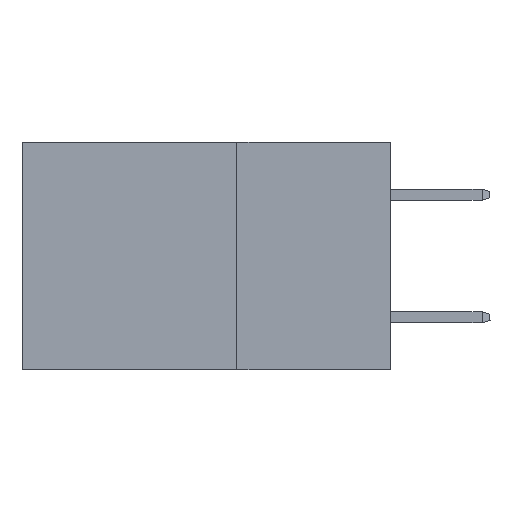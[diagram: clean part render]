
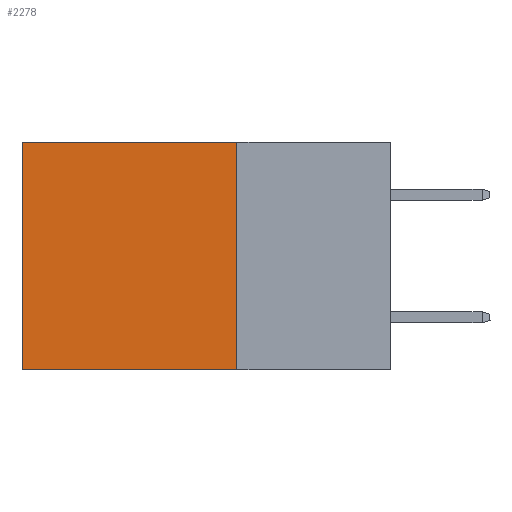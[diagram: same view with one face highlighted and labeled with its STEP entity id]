
A CAD part, left-side view. The second image highlights one B-rep face of the part: STEP entity #2278.
In plain terms, the highlighted planar face has unit normal (-1, 0, 0).
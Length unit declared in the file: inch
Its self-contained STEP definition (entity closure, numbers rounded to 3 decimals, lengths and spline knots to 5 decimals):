
#25 = LINE ( 'NONE', #17002, #10914 ) ;
#1154 = DIRECTION ( 'NONE',  ( 0., 1., 0. ) ) ;
#2278 = ADVANCED_FACE ( 'NONE', ( #18125 ), #16090, .F. ) ;
#2668 = CARTESIAN_POINT ( 'NONE',  ( 0.2875, 0.25, 0. ) ) ;
#3081 = VECTOR ( 'NONE', #5774, 39.37008 ) ;
#5774 = DIRECTION ( 'NONE',  ( 0., 0., -1. ) ) ;
#6467 = VECTOR ( 'NONE', #13831, 39.37008 ) ;
#6862 = VERTEX_POINT ( 'NONE', #9644 ) ;
#7752 = VERTEX_POINT ( 'NONE', #12504 ) ;
#8001 = LINE ( 'NONE', #8198, #10917 ) ;
#8198 = CARTESIAN_POINT ( 'NONE',  ( 0.2875, 0.25, 0. ) ) ;
#8431 = DIRECTION ( 'NONE',  ( 0., 1., 0. ) ) ;
#9117 = EDGE_CURVE ( 'NONE', #13216, #7752, #13255, .T. ) ;
#9223 = EDGE_CURVE ( 'NONE', #13216, #11601, #8001, .T. ) ;
#9644 = CARTESIAN_POINT ( 'NONE',  ( 0.2875, 0.6, -0.37 ) ) ;
#10241 = DIRECTION ( 'NONE',  ( 0., 0., -1. ) ) ;
#10796 = AXIS2_PLACEMENT_3D ( 'NONE', #14763, #11859, #10241 ) ;
#10914 = VECTOR ( 'NONE', #1154, 39.37008 ) ;
#10917 = VECTOR ( 'NONE', #8431, 39.37008 ) ;
#11028 = CARTESIAN_POINT ( 'NONE',  ( 0.2875, 0.25, 0. ) ) ;
#11566 = EDGE_LOOP ( 'NONE', ( #13420, #16666, #16898, #16736 ) ) ;
#11601 = VERTEX_POINT ( 'NONE', #13120 ) ;
#11859 = DIRECTION ( 'NONE',  ( 1., 0., 0. ) ) ;
#12504 = CARTESIAN_POINT ( 'NONE',  ( 0.2875, 0.25, -0.37 ) ) ;
#13120 = CARTESIAN_POINT ( 'NONE',  ( 0.2875, 0.6, 0. ) ) ;
#13216 = VERTEX_POINT ( 'NONE', #2668 ) ;
#13255 = LINE ( 'NONE', #11028, #6467 ) ;
#13420 = ORIENTED_EDGE ( 'NONE', *, *, #15662, .T. ) ;
#13831 = DIRECTION ( 'NONE',  ( 0., 0., -1. ) ) ;
#14763 = CARTESIAN_POINT ( 'NONE',  ( 0.2875, 0.25, 0. ) ) ;
#15495 = CARTESIAN_POINT ( 'NONE',  ( 0.2875, 0.6, 0. ) ) ;
#15662 = EDGE_CURVE ( 'NONE', #11601, #6862, #17781, .T. ) ;
#16090 = PLANE ( 'NONE',  #10796 ) ;
#16666 = ORIENTED_EDGE ( 'NONE', *, *, #17763, .F. ) ;
#16736 = ORIENTED_EDGE ( 'NONE', *, *, #9223, .T. ) ;
#16898 = ORIENTED_EDGE ( 'NONE', *, *, #9117, .F. ) ;
#17002 = CARTESIAN_POINT ( 'NONE',  ( 0.2875, 0.25, -0.37 ) ) ;
#17763 = EDGE_CURVE ( 'NONE', #7752, #6862, #25, .T. ) ;
#17781 = LINE ( 'NONE', #15495, #3081 ) ;
#18125 = FACE_OUTER_BOUND ( 'NONE', #11566, .T. ) ;
